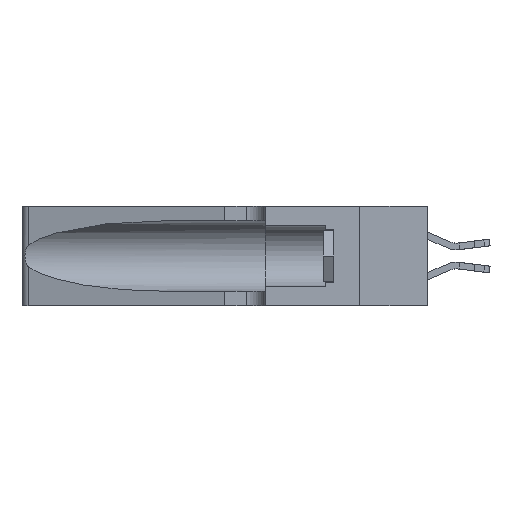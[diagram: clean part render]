
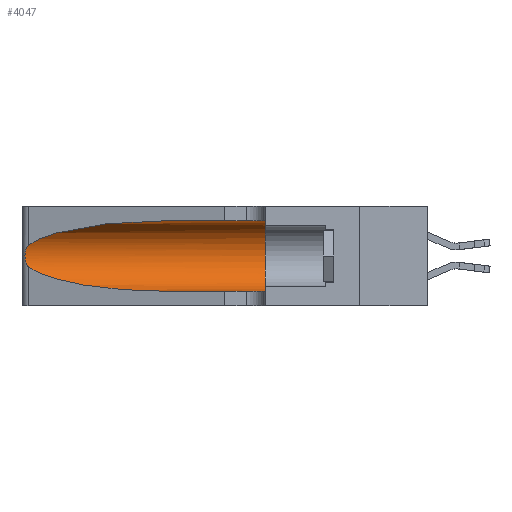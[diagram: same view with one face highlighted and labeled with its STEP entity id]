
A CAD part, left-side view. The second image highlights one B-rep face of the part: STEP entity #4047.
In plain terms, the highlighted cylindrical face has radius 3.308 mm (diameter 6.617 mm), a partial arc.
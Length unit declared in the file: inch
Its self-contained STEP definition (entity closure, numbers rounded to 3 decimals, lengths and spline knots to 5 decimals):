
#626 = CARTESIAN_POINT ( 'NONE',  ( 0.25487, 1.22718, 0.14631 ) ) ;
#1074 = CARTESIAN_POINT ( 'NONE',  ( 0.1305, 1.61858, 0.05475 ) ) ;
#1180 = CARTESIAN_POINT ( 'NONE',  ( 0.2373, 1.15595, 0.28018 ) ) ;
#1215 = CARTESIAN_POINT ( 'NONE',  ( 0.25854, 1.2359, 0.20912 ) ) ;
#1695 =( BOUNDED_CURVE ( )  B_SPLINE_CURVE ( 3, ( #3020, #23071, #1180, #14155 ),
 .UNSPECIFIED., .F., .T. ) 
 B_SPLINE_CURVE_WITH_KNOTS ( ( 4, 4 ),
 ( 1.5708, 2.84003 ),
 .UNSPECIFIED. ) 
 CURVE ( )  GEOMETRIC_REPRESENTATION_ITEM ( )  RATIONAL_B_SPLINE_CURVE ( ( 1., 0.87, 0.87, 1. ) ) 
 REPRESENTATION_ITEM ( '' )  );
#2164 = CARTESIAN_POINT ( 'NONE',  ( 0.25487, 1.22718, 0.22369 ) ) ;
#2211 = CARTESIAN_POINT ( 'NONE',  ( 0.1305, 0.72297, 0.31525 ) ) ;
#2911 = CARTESIAN_POINT ( 'NONE',  ( 0.1305, 0.72297, 0.05475 ) ) ;
#3020 = CARTESIAN_POINT ( 'NONE',  ( 0.1305, 0.72297, 0.31525 ) ) ;
#3045 = CARTESIAN_POINT ( 'NONE',  ( 0.25487, 1.22718, 0.14631 ) ) ;
#3132 = CARTESIAN_POINT ( 'NONE',  ( 0.26075, 1.23896, 0.19203 ) ) ;
#3171 = ORIENTED_EDGE ( 'NONE', *, *, #20894, .T. ) ;
#3965 = VERTEX_POINT ( 'NONE', #15258 ) ;
#4047 = ADVANCED_FACE ( 'NONE', ( #8121 ), #7533, .F. ) ;
#4059 = ORIENTED_EDGE ( 'NONE', *, *, #5468, .T. ) ;
#5017 = CARTESIAN_POINT ( 'NONE',  ( 0.26017, 1.23833, 0.17102 ) ) ;
#5381 = DIRECTION ( 'NONE',  ( 0., 1., 0. ) ) ;
#5468 = EDGE_CURVE ( 'NONE', #8866, #21041, #1695, .T. ) ;
#6273 = DIRECTION ( 'NONE',  ( 0., 0., -1. ) ) ;
#6662 = EDGE_LOOP ( 'NONE', ( #4059, #3171, #9271, #20089, #18100, #14807 ) ) ;
#6885 = CARTESIAN_POINT ( 'NONE',  ( 0.25789, 1.23486, 0.15765 ) ) ;
#7384 = EDGE_CURVE ( 'NONE', #3965, #9164, #19617, .T. ) ;
#7533 = CYLINDRICAL_SURFACE ( 'NONE', #10225, 0.13025 ) ;
#8121 = FACE_OUTER_BOUND ( 'NONE', #6662, .T. ) ;
#8419 = EDGE_CURVE ( 'NONE', #12383, #20218, #17067, .T. ) ;
#8744 = CARTESIAN_POINT ( 'NONE',  ( 0.25555, 1.22993, 0.14849 ) ) ;
#8866 = VERTEX_POINT ( 'NONE', #2211 ) ;
#9164 = VERTEX_POINT ( 'NONE', #23144 ) ;
#9271 = ORIENTED_EDGE ( 'NONE', *, *, #8419, .T. ) ;
#9952 = CARTESIAN_POINT ( 'NONE',  ( 0.18966, 0.96281, 0.05475 ) ) ;
#10225 = AXIS2_PLACEMENT_3D ( 'NONE', #19031, #11864, #6273 ) ;
#11864 = DIRECTION ( 'NONE',  ( 0., -1., 0. ) ) ;
#12264 = DIRECTION ( 'NONE',  ( 0., -1., 0. ) ) ;
#12383 = VERTEX_POINT ( 'NONE', #3045 ) ;
#12395 = CARTESIAN_POINT ( 'NONE',  ( 0.25787, 1.23484, 0.2124 ) ) ;
#12576 = LINE ( 'NONE', #21559, #22127 ) ;
#13650 = CARTESIAN_POINT ( 'NONE',  ( 0.1305, 0.72297, 0.05475 ) ) ;
#14155 = CARTESIAN_POINT ( 'NONE',  ( 0.25487, 1.22718, 0.22369 ) ) ;
#14195 = CARTESIAN_POINT ( 'NONE',  ( 0.26018, 1.23835, 0.19895 ) ) ;
#14807 = ORIENTED_EDGE ( 'NONE', *, *, #19746, .F. ) ;
#15258 = CARTESIAN_POINT ( 'NONE',  ( 0.1305, 0.35, 0.31525 ) ) ;
#15756 = VECTOR ( 'NONE', #12264, 39.37008 ) ;
#16010 = CARTESIAN_POINT ( 'NONE',  ( 0.26075, 1.23896, 0.178 ) ) ;
#16319 = LINE ( 'NONE', #1074, #15756 ) ;
#16367 = CARTESIAN_POINT ( 'NONE',  ( 0.1305, 0.35, 0.185 ) ) ;
#17067 =( BOUNDED_CURVE ( )  B_SPLINE_CURVE ( 3, ( #626, #22589, #9952, #13650 ),
 .UNSPECIFIED., .F., .F. ) 
 B_SPLINE_CURVE_WITH_KNOTS ( ( 4, 4 ),
 ( 3.44316, 4.71239 ),
 .UNSPECIFIED. ) 
 CURVE ( )  GEOMETRIC_REPRESENTATION_ITEM ( )  RATIONAL_B_SPLINE_CURVE ( ( 1., 0.87, 0.87, 1. ) ) 
 REPRESENTATION_ITEM ( '' )  );
#17389 = EDGE_CURVE ( 'NONE', #20218, #9164, #16319, .T. ) ;
#17803 = CARTESIAN_POINT ( 'NONE',  ( 0.25856, 1.23593, 0.16098 ) ) ;
#18100 = ORIENTED_EDGE ( 'NONE', *, *, #7384, .F. ) ;
#18166 = DIRECTION ( 'NONE',  ( 0., 0., 1. ) ) ;
#19031 = CARTESIAN_POINT ( 'NONE',  ( 0.1305, 1.61858, 0.185 ) ) ;
#19559 = CARTESIAN_POINT ( 'NONE',  ( 0.25555, 1.22994, 0.2215 ) ) ;
#19617 = CIRCLE ( 'NONE', #21069, 0.13025 ) ;
#19632 = CARTESIAN_POINT ( 'NONE',  ( 0.25639, 1.23186, 0.15144 ) ) ;
#19746 = EDGE_CURVE ( 'NONE', #8866, #3965, #12576, .T. ) ;
#20089 = ORIENTED_EDGE ( 'NONE', *, *, #17389, .T. ) ;
#20218 = VERTEX_POINT ( 'NONE', #2911 ) ;
#20894 = EDGE_CURVE ( 'NONE', #21041, #12383, #21944, .T. ) ;
#21041 = VERTEX_POINT ( 'NONE', #2164 ) ;
#21069 = AXIS2_PLACEMENT_3D ( 'NONE', #16367, #5381, #18166 ) ;
#21355 = CARTESIAN_POINT ( 'NONE',  ( 0.25487, 1.22718, 0.22369 ) ) ;
#21432 = CARTESIAN_POINT ( 'NONE',  ( 0.25487, 1.22718, 0.14631 ) ) ;
#21559 = CARTESIAN_POINT ( 'NONE',  ( 0.1305, 1.61858, 0.31525 ) ) ;
#21944 = B_SPLINE_CURVE_WITH_KNOTS ( 'NONE', 3,
 ( #21355, #19559, #23103, #12395, #1215, #14195, #3132, #16010, #5017, #17803, #6885, #19632, #8744, #21432 ),
 .UNSPECIFIED., .F., .F.,
 ( 4, 2, 2, 2, 2, 2, 4 ),
 ( 0., 0.00027, 0.00053, 0.00107, 0.0016, 0.00187, 0.00214 ),
 .UNSPECIFIED. ) ;
#22127 = VECTOR ( 'NONE', #23309, 39.37008 ) ;
#22589 = CARTESIAN_POINT ( 'NONE',  ( 0.2373, 1.15595, 0.08982 ) ) ;
#23071 = CARTESIAN_POINT ( 'NONE',  ( 0.18966, 0.96281, 0.31525 ) ) ;
#23103 = CARTESIAN_POINT ( 'NONE',  ( 0.25639, 1.23184, 0.21858 ) ) ;
#23144 = CARTESIAN_POINT ( 'NONE',  ( 0.1305, 0.35, 0.05475 ) ) ;
#23309 = DIRECTION ( 'NONE',  ( 0., -1., 0. ) ) ;
